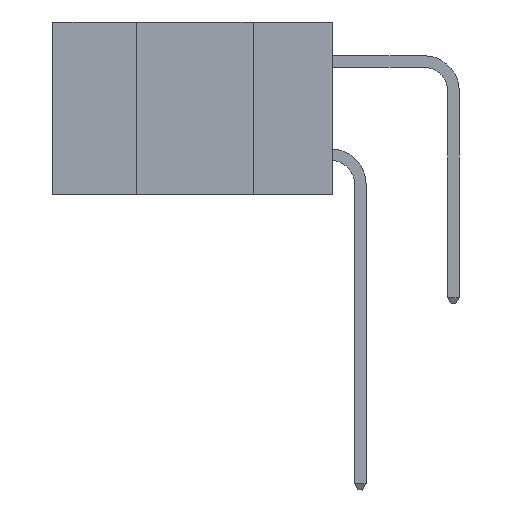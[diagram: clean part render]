
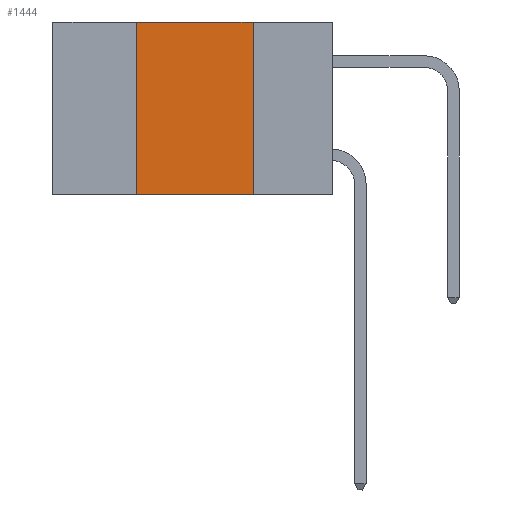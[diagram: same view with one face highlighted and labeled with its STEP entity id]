
A CAD part, left-side view. The second image highlights one B-rep face of the part: STEP entity #1444.
In plain terms, the highlighted planar face has unit normal (-1, 0, 0).
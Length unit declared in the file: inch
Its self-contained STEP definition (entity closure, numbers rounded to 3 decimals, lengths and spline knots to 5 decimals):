
#667 = VECTOR ( 'NONE', #9885, 39.37008 ) ;
#681 = EDGE_LOOP ( 'NONE', ( #1917, #15980, #1311, #8346 ) ) ;
#839 = EDGE_CURVE ( 'NONE', #16185, #2670, #14245, .T. ) ;
#1311 = ORIENTED_EDGE ( 'NONE', *, *, #2416, .F. ) ;
#1444 = ADVANCED_FACE ( 'NONE', ( #3646 ), #4357, .F. ) ;
#1917 = ORIENTED_EDGE ( 'NONE', *, *, #15182, .F. ) ;
#2416 = EDGE_CURVE ( 'NONE', #16185, #7991, #7632, .T. ) ;
#2670 = VERTEX_POINT ( 'NONE', #12595 ) ;
#3041 = EDGE_CURVE ( 'NONE', #7991, #4942, #3680, .T. ) ;
#3646 = FACE_OUTER_BOUND ( 'NONE', #681, .T. ) ;
#3680 = LINE ( 'NONE', #8716, #6929 ) ;
#3714 = VECTOR ( 'NONE', #5236, 39.37008 ) ;
#4357 = PLANE ( 'NONE',  #14054 ) ;
#4942 = VERTEX_POINT ( 'NONE', #8395 ) ;
#5236 = DIRECTION ( 'NONE',  ( 0., 0., 1. ) ) ;
#6415 = CARTESIAN_POINT ( 'NONE',  ( 0., 0.17, 0. ) ) ;
#6618 = CARTESIAN_POINT ( 'NONE',  ( 0., 0.42, -0.37 ) ) ;
#6929 = VECTOR ( 'NONE', #16219, 39.37008 ) ;
#7553 = LINE ( 'NONE', #6415, #16266 ) ;
#7632 = LINE ( 'NONE', #18341, #3714 ) ;
#7858 = DIRECTION ( 'NONE',  ( 0., 0., -1. ) ) ;
#7991 = VERTEX_POINT ( 'NONE', #14129 ) ;
#8346 = ORIENTED_EDGE ( 'NONE', *, *, #839, .T. ) ;
#8395 = CARTESIAN_POINT ( 'NONE',  ( 0., 0.17, 0. ) ) ;
#8716 = CARTESIAN_POINT ( 'NONE',  ( 0., 0.6, 0. ) ) ;
#8786 = DIRECTION ( 'NONE',  ( 1., 0., 0. ) ) ;
#9885 = DIRECTION ( 'NONE',  ( 0., -1., 0. ) ) ;
#12595 = CARTESIAN_POINT ( 'NONE',  ( 0., 0.17, -0.37 ) ) ;
#14054 = AXIS2_PLACEMENT_3D ( 'NONE', #17545, #8786, #17600 ) ;
#14129 = CARTESIAN_POINT ( 'NONE',  ( 0., 0.42, 0. ) ) ;
#14245 = LINE ( 'NONE', #14314, #667 ) ;
#14314 = CARTESIAN_POINT ( 'NONE',  ( 0., 0.6, -0.37 ) ) ;
#15182 = EDGE_CURVE ( 'NONE', #4942, #2670, #7553, .T. ) ;
#15980 = ORIENTED_EDGE ( 'NONE', *, *, #3041, .F. ) ;
#16185 = VERTEX_POINT ( 'NONE', #6618 ) ;
#16219 = DIRECTION ( 'NONE',  ( 0., -1., 0. ) ) ;
#16266 = VECTOR ( 'NONE', #7858, 39.37008 ) ;
#17545 = CARTESIAN_POINT ( 'NONE',  ( 0., 0.6, 0. ) ) ;
#17600 = DIRECTION ( 'NONE',  ( 0., 0., -1. ) ) ;
#18341 = CARTESIAN_POINT ( 'NONE',  ( 0., 0.42, 0. ) ) ;
